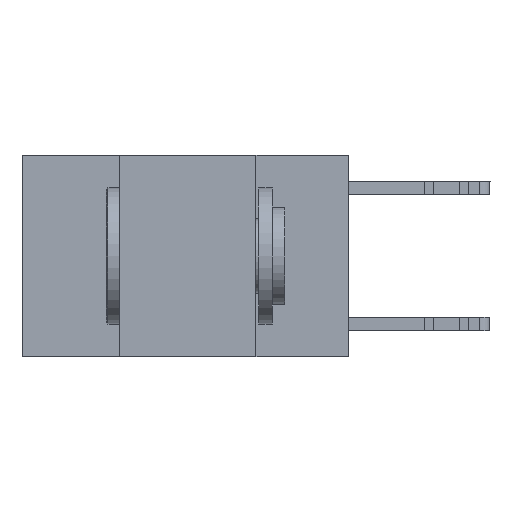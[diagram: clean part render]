
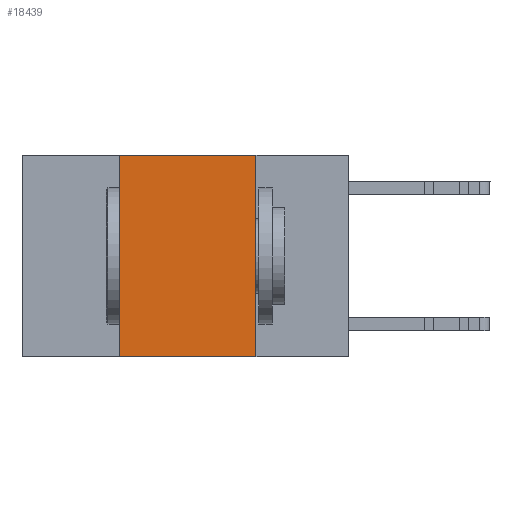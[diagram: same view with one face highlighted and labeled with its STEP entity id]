
A CAD part, left-side view. The second image highlights one B-rep face of the part: STEP entity #18439.
In plain terms, the highlighted planar face has unit normal (-1, 0, 0).
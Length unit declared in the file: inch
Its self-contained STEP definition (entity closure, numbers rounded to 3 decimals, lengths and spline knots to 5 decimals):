
#438 = ORIENTED_EDGE ( 'NONE', *, *, #2857, .F. ) ;
#1269 = DIRECTION ( 'NONE',  ( 0., -1., 0. ) ) ;
#1989 = EDGE_CURVE ( 'NONE', #8863, #9275, #20703, .T. ) ;
#2857 = EDGE_CURVE ( 'NONE', #25956, #8863, #9283, .T. ) ;
#2865 = EDGE_LOOP ( 'NONE', ( #23235, #438, #18904, #4498 ) ) ;
#3665 = CARTESIAN_POINT ( 'NONE',  ( 0., 0.17, 0. ) ) ;
#3933 = DIRECTION ( 'NONE',  ( 0., -1., 0. ) ) ;
#4289 = LINE ( 'NONE', #17595, #7304 ) ;
#4498 = ORIENTED_EDGE ( 'NONE', *, *, #12626, .T. ) ;
#5777 = LINE ( 'NONE', #26601, #15587 ) ;
#5853 = EDGE_CURVE ( 'NONE', #15313, #25956, #4289, .T. ) ;
#7304 = VECTOR ( 'NONE', #13395, 39.37008 ) ;
#8863 = VERTEX_POINT ( 'NONE', #3665 ) ;
#9275 = VERTEX_POINT ( 'NONE', #18893 ) ;
#9283 = LINE ( 'NONE', #27551, #24997 ) ;
#11728 = CARTESIAN_POINT ( 'NONE',  ( 0., 0.17, 0. ) ) ;
#12626 = EDGE_CURVE ( 'NONE', #15313, #9275, #5777, .T. ) ;
#13395 = DIRECTION ( 'NONE',  ( 0., 0., 1. ) ) ;
#13526 = FACE_OUTER_BOUND ( 'NONE', #2865, .T. ) ;
#13944 = CARTESIAN_POINT ( 'NONE',  ( 0., 0.42, -0.37 ) ) ;
#15313 = VERTEX_POINT ( 'NONE', #13944 ) ;
#15587 = VECTOR ( 'NONE', #1269, 39.37008 ) ;
#17595 = CARTESIAN_POINT ( 'NONE',  ( 0., 0.42, 0. ) ) ;
#18439 = ADVANCED_FACE ( 'NONE', ( #13526 ), #20272, .F. ) ;
#18893 = CARTESIAN_POINT ( 'NONE',  ( 0., 0.17, -0.37 ) ) ;
#18904 = ORIENTED_EDGE ( 'NONE', *, *, #5853, .F. ) ;
#20043 = AXIS2_PLACEMENT_3D ( 'NONE', #22660, #29151, #20955 ) ;
#20272 = PLANE ( 'NONE',  #20043 ) ;
#20703 = LINE ( 'NONE', #11728, #20936 ) ;
#20936 = VECTOR ( 'NONE', #25691, 39.37008 ) ;
#20955 = DIRECTION ( 'NONE',  ( 0., 0., -1. ) ) ;
#22404 = CARTESIAN_POINT ( 'NONE',  ( 0., 0.42, 0. ) ) ;
#22660 = CARTESIAN_POINT ( 'NONE',  ( 0., 0.6, 0. ) ) ;
#23235 = ORIENTED_EDGE ( 'NONE', *, *, #1989, .F. ) ;
#24997 = VECTOR ( 'NONE', #3933, 39.37008 ) ;
#25691 = DIRECTION ( 'NONE',  ( 0., 0., -1. ) ) ;
#25956 = VERTEX_POINT ( 'NONE', #22404 ) ;
#26601 = CARTESIAN_POINT ( 'NONE',  ( 0., 0.6, -0.37 ) ) ;
#27551 = CARTESIAN_POINT ( 'NONE',  ( 0., 0.6, 0. ) ) ;
#29151 = DIRECTION ( 'NONE',  ( 1., 0., 0. ) ) ;
